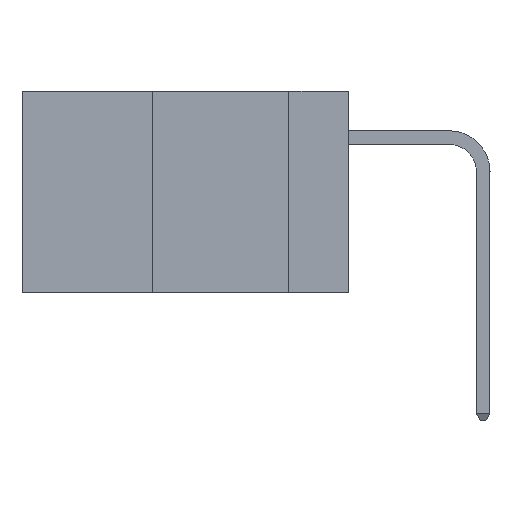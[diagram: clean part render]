
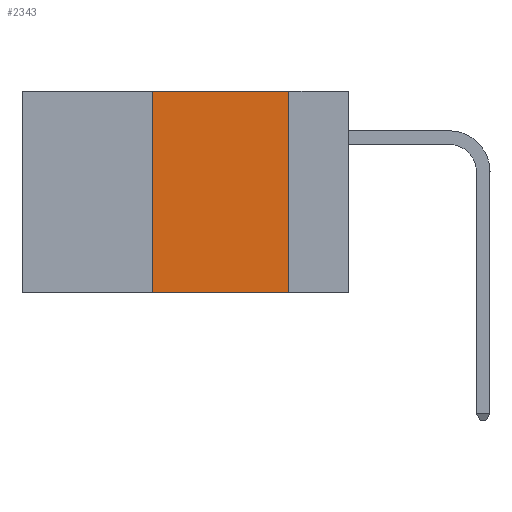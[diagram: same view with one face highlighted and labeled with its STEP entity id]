
A CAD part, left-side view. The second image highlights one B-rep face of the part: STEP entity #2343.
In plain terms, the highlighted planar face has unit normal (-1, 0, 0).
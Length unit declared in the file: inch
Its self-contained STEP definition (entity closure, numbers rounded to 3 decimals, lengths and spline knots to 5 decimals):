
#1380 = VERTEX_POINT ( 'NONE', #8225 ) ;
#2343 = ADVANCED_FACE ( 'NONE', ( #23164 ), #14329, .F. ) ;
#2765 = ORIENTED_EDGE ( 'NONE', *, *, #5881, .F. ) ;
#3348 = DIRECTION ( 'NONE',  ( 1., 0., 0. ) ) ;
#4565 = DIRECTION ( 'NONE',  ( 0., -1., 0. ) ) ;
#5881 = EDGE_CURVE ( 'NONE', #15444, #1380, #40094, .T. ) ;
#8071 = VECTOR ( 'NONE', #8990, 39.37008 ) ;
#8225 = CARTESIAN_POINT ( 'NONE',  ( 0., 0.11, 0. ) ) ;
#8990 = DIRECTION ( 'NONE',  ( 0., -1., 0. ) ) ;
#12156 = CARTESIAN_POINT ( 'NONE',  ( 0., 0.6, 0. ) ) ;
#14329 = PLANE ( 'NONE',  #18367 ) ;
#14370 = LINE ( 'NONE', #45688, #8071 ) ;
#14428 = ORIENTED_EDGE ( 'NONE', *, *, #18689, .F. ) ;
#14444 = CARTESIAN_POINT ( 'NONE',  ( 0., 0.11, 0. ) ) ;
#15444 = VERTEX_POINT ( 'NONE', #18080 ) ;
#16864 = ORIENTED_EDGE ( 'NONE', *, *, #18470, .F. ) ;
#17089 = VECTOR ( 'NONE', #38408, 39.37008 ) ;
#18080 = CARTESIAN_POINT ( 'NONE',  ( 0., 0.36, 0. ) ) ;
#18367 = AXIS2_PLACEMENT_3D ( 'NONE', #40200, #3348, #29410 ) ;
#18470 = EDGE_CURVE ( 'NONE', #35228, #15444, #37926, .T. ) ;
#18689 = EDGE_CURVE ( 'NONE', #1380, #34383, #35570, .T. ) ;
#19746 = ORIENTED_EDGE ( 'NONE', *, *, #21171, .T. ) ;
#20064 = CARTESIAN_POINT ( 'NONE',  ( 0., 0.11, -0.37 ) ) ;
#21171 = EDGE_CURVE ( 'NONE', #35228, #34383, #14370, .T. ) ;
#23164 = FACE_OUTER_BOUND ( 'NONE', #41939, .T. ) ;
#24496 = VECTOR ( 'NONE', #4565, 39.37008 ) ;
#25739 = VECTOR ( 'NONE', #32274, 39.37008 ) ;
#28075 = CARTESIAN_POINT ( 'NONE',  ( 0., 0.36, -0.37 ) ) ;
#29410 = DIRECTION ( 'NONE',  ( 0., 0., -1. ) ) ;
#32274 = DIRECTION ( 'NONE',  ( 0., 0., -1. ) ) ;
#34383 = VERTEX_POINT ( 'NONE', #20064 ) ;
#35228 = VERTEX_POINT ( 'NONE', #28075 ) ;
#35570 = LINE ( 'NONE', #14444, #25739 ) ;
#37926 = LINE ( 'NONE', #38565, #17089 ) ;
#38408 = DIRECTION ( 'NONE',  ( 0., 0., 1. ) ) ;
#38565 = CARTESIAN_POINT ( 'NONE',  ( 0., 0.36, 0. ) ) ;
#40094 = LINE ( 'NONE', #12156, #24496 ) ;
#40200 = CARTESIAN_POINT ( 'NONE',  ( 0., 0.6, 0. ) ) ;
#41939 = EDGE_LOOP ( 'NONE', ( #14428, #2765, #16864, #19746 ) ) ;
#45688 = CARTESIAN_POINT ( 'NONE',  ( 0., 0.6, -0.37 ) ) ;
